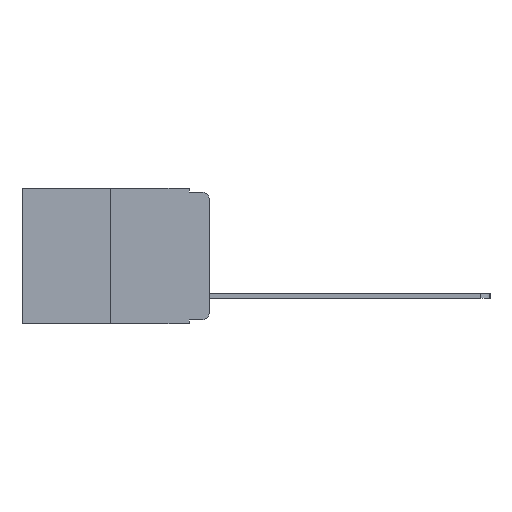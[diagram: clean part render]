
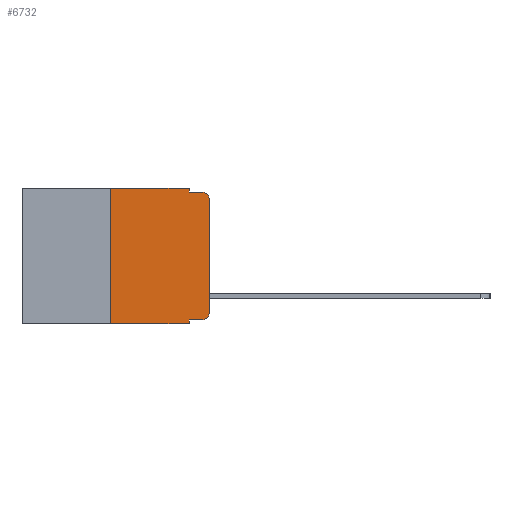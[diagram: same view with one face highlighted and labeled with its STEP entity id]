
A CAD part, left-side view. The second image highlights one B-rep face of the part: STEP entity #6732.
In plain terms, the highlighted planar face has unit normal (-1, 0, 0).
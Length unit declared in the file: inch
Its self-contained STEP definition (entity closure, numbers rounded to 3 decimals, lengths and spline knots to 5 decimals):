
#270 = CARTESIAN_POINT ( 'NONE',  ( 0., 0., -0.03 ) ) ;
#860 = CARTESIAN_POINT ( 'NONE',  ( 0., 0.051, 0. ) ) ;
#911 = VERTEX_POINT ( 'NONE', #13840 ) ;
#912 = DIRECTION ( 'NONE',  ( 0., 0., -1. ) ) ;
#980 = EDGE_CURVE ( 'NONE', #4263, #16211, #14030, .T. ) ;
#1945 = ORIENTED_EDGE ( 'NONE', *, *, #980, .F. ) ;
#1997 = VECTOR ( 'NONE', #912, 39.37008 ) ;
#2085 = EDGE_CURVE ( 'NONE', #17424, #16650, #18132, .T. ) ;
#2278 = CARTESIAN_POINT ( 'NONE',  ( 0., 0.25, -0.343 ) ) ;
#2292 = VECTOR ( 'NONE', #7377, 39.37008 ) ;
#2360 = VECTOR ( 'NONE', #2745, 39.37008 ) ;
#2460 = CARTESIAN_POINT ( 'NONE',  ( 0., 0.051, 0. ) ) ;
#2745 = DIRECTION ( 'NONE',  ( 0., 0., -1. ) ) ;
#2818 = LINE ( 'NONE', #10082, #18116 ) ;
#3040 = VERTEX_POINT ( 'NONE', #270 ) ;
#3224 = EDGE_CURVE ( 'NONE', #13221, #9152, #13274, .T. ) ;
#3251 = CARTESIAN_POINT ( 'NONE',  ( 0., 0.051, 0. ) ) ;
#3638 = LINE ( 'NONE', #6096, #18785 ) ;
#3812 = LINE ( 'NONE', #14501, #18911 ) ;
#4263 = VERTEX_POINT ( 'NONE', #16431 ) ;
#4308 = CARTESIAN_POINT ( 'NONE',  ( 0., 0., 0. ) ) ;
#4363 = EDGE_LOOP ( 'NONE', ( #7417, #11172, #18462, #9901, #5168, #14309, #10088, #1945, #4492, #10306 ) ) ;
#4492 = ORIENTED_EDGE ( 'NONE', *, *, #17488, .T. ) ;
#5168 = ORIENTED_EDGE ( 'NONE', *, *, #12199, .F. ) ;
#5367 = EDGE_CURVE ( 'NONE', #9152, #911, #3638, .T. ) ;
#5410 = DIRECTION ( 'NONE',  ( 0., -1., 0. ) ) ;
#5871 = VECTOR ( 'NONE', #5884, 39.37008 ) ;
#5884 = DIRECTION ( 'NONE',  ( 0., 0., 1. ) ) ;
#6057 = CIRCLE ( 'NONE', #14428, 0.02 ) ;
#6087 = VECTOR ( 'NONE', #15642, 39.37008 ) ;
#6096 = CARTESIAN_POINT ( 'NONE',  ( 0., 0.051, -0.01 ) ) ;
#6601 = LINE ( 'NONE', #8471, #6087 ) ;
#6732 = ADVANCED_FACE ( 'NONE', ( #8815 ), #12260, .F. ) ;
#7377 = DIRECTION ( 'NONE',  ( 0., 0., 1. ) ) ;
#7417 = ORIENTED_EDGE ( 'NONE', *, *, #15251, .T. ) ;
#7570 = CARTESIAN_POINT ( 'NONE',  ( 0., 0.25, 0. ) ) ;
#7708 = DIRECTION ( 'NONE',  ( 0., -1., 0. ) ) ;
#8237 = CIRCLE ( 'NONE', #11326, 0.02 ) ;
#8448 = DIRECTION ( 'NONE',  ( -1., 0., 0. ) ) ;
#8471 = CARTESIAN_POINT ( 'NONE',  ( 0., 0.473, -0.343 ) ) ;
#8528 = CARTESIAN_POINT ( 'NONE',  ( 0., 0., -0.313 ) ) ;
#8773 = DIRECTION ( 'NONE',  ( -1., 0., 0. ) ) ;
#8815 = FACE_OUTER_BOUND ( 'NONE', #4363, .T. ) ;
#9152 = VERTEX_POINT ( 'NONE', #15395 ) ;
#9293 = VERTEX_POINT ( 'NONE', #8528 ) ;
#9413 = DIRECTION ( 'NONE',  ( 0., 0., -1. ) ) ;
#9901 = ORIENTED_EDGE ( 'NONE', *, *, #3224, .F. ) ;
#10082 = CARTESIAN_POINT ( 'NONE',  ( 0., 0.473, 0. ) ) ;
#10088 = ORIENTED_EDGE ( 'NONE', *, *, #11694, .T. ) ;
#10306 = ORIENTED_EDGE ( 'NONE', *, *, #16538, .T. ) ;
#11095 = AXIS2_PLACEMENT_3D ( 'NONE', #15104, #17924, #9413 ) ;
#11172 = ORIENTED_EDGE ( 'NONE', *, *, #14330, .T. ) ;
#11326 = AXIS2_PLACEMENT_3D ( 'NONE', #17324, #8773, #18708 ) ;
#11694 = EDGE_CURVE ( 'NONE', #17424, #16211, #6601, .T. ) ;
#12199 = EDGE_CURVE ( 'NONE', #16650, #13221, #2818, .T. ) ;
#12260 = PLANE ( 'NONE',  #11095 ) ;
#13221 = VERTEX_POINT ( 'NONE', #2460 ) ;
#13274 = LINE ( 'NONE', #860, #1997 ) ;
#13840 = CARTESIAN_POINT ( 'NONE',  ( 0., 0.02, -0.01 ) ) ;
#14030 = LINE ( 'NONE', #3251, #2360 ) ;
#14098 = CARTESIAN_POINT ( 'NONE',  ( 0., 0.02, -0.333 ) ) ;
#14309 = ORIENTED_EDGE ( 'NONE', *, *, #2085, .F. ) ;
#14330 = EDGE_CURVE ( 'NONE', #3040, #911, #8237, .T. ) ;
#14395 = CARTESIAN_POINT ( 'NONE',  ( 0., 0.25, 0. ) ) ;
#14428 = AXIS2_PLACEMENT_3D ( 'NONE', #17010, #8448, #18433 ) ;
#14501 = CARTESIAN_POINT ( 'NONE',  ( 0., 0.051, -0.333 ) ) ;
#14669 = LINE ( 'NONE', #4308, #5871 ) ;
#15104 = CARTESIAN_POINT ( 'NONE',  ( 0., 0.473, 0. ) ) ;
#15251 = EDGE_CURVE ( 'NONE', #9293, #3040, #14669, .T. ) ;
#15395 = CARTESIAN_POINT ( 'NONE',  ( 0., 0.051, -0.01 ) ) ;
#15642 = DIRECTION ( 'NONE',  ( 0., -1., 0. ) ) ;
#16211 = VERTEX_POINT ( 'NONE', #19177 ) ;
#16431 = CARTESIAN_POINT ( 'NONE',  ( 0., 0.051, -0.333 ) ) ;
#16538 = EDGE_CURVE ( 'NONE', #18505, #9293, #6057, .T. ) ;
#16650 = VERTEX_POINT ( 'NONE', #14395 ) ;
#17010 = CARTESIAN_POINT ( 'NONE',  ( 0., 0.02, -0.313 ) ) ;
#17301 = DIRECTION ( 'NONE',  ( 0., -1., 0. ) ) ;
#17324 = CARTESIAN_POINT ( 'NONE',  ( 0., 0.02, -0.03 ) ) ;
#17424 = VERTEX_POINT ( 'NONE', #2278 ) ;
#17488 = EDGE_CURVE ( 'NONE', #4263, #18505, #3812, .T. ) ;
#17924 = DIRECTION ( 'NONE',  ( 1., 0., 0. ) ) ;
#18116 = VECTOR ( 'NONE', #5410, 39.37008 ) ;
#18132 = LINE ( 'NONE', #7570, #2292 ) ;
#18433 = DIRECTION ( 'NONE',  ( 0., 0., -1. ) ) ;
#18462 = ORIENTED_EDGE ( 'NONE', *, *, #5367, .F. ) ;
#18505 = VERTEX_POINT ( 'NONE', #14098 ) ;
#18708 = DIRECTION ( 'NONE',  ( 0., 0., -1. ) ) ;
#18785 = VECTOR ( 'NONE', #7708, 39.37008 ) ;
#18911 = VECTOR ( 'NONE', #17301, 39.37008 ) ;
#19177 = CARTESIAN_POINT ( 'NONE',  ( 0., 0.051, -0.343 ) ) ;
